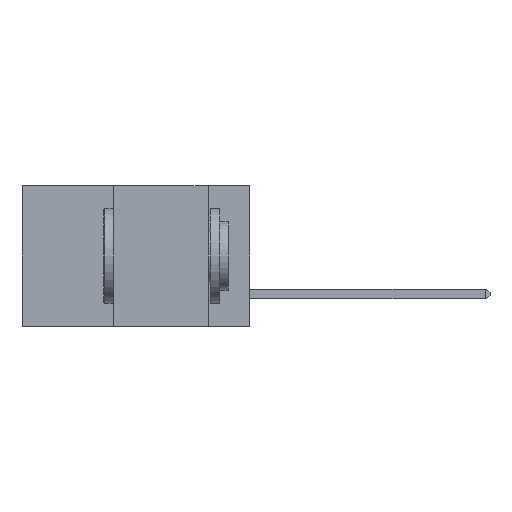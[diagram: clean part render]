
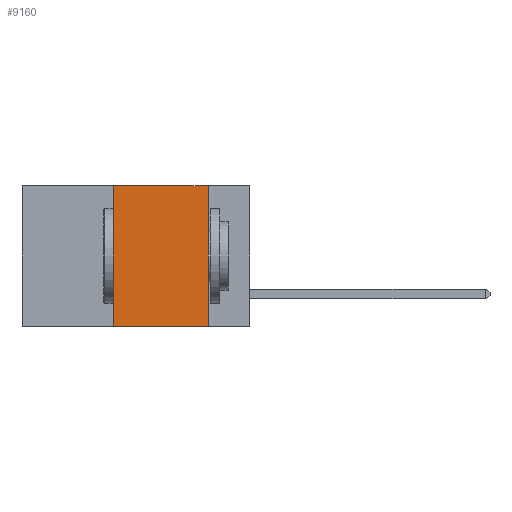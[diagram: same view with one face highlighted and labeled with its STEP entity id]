
A CAD part, left-side view. The second image highlights one B-rep face of the part: STEP entity #9160.
In plain terms, the highlighted planar face has unit normal (-1, 0, 0).
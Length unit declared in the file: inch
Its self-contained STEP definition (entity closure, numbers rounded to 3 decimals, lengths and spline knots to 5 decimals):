
#709 = CARTESIAN_POINT ( 'NONE',  ( 0., 0.6, 0. ) ) ;
#1688 = DIRECTION ( 'NONE',  ( 0., -1., 0. ) ) ;
#2287 = CARTESIAN_POINT ( 'NONE',  ( 0., 0.11, 0. ) ) ;
#3068 = PLANE ( 'NONE',  #20363 ) ;
#3190 = VERTEX_POINT ( 'NONE', #6400 ) ;
#3540 = EDGE_CURVE ( 'NONE', #4156, #19427, #22852, .T. ) ;
#3720 = CARTESIAN_POINT ( 'NONE',  ( 0., 0.11, 0. ) ) ;
#4156 = VERTEX_POINT ( 'NONE', #3720 ) ;
#4837 = LINE ( 'NONE', #22997, #25956 ) ;
#4890 = EDGE_CURVE ( 'NONE', #3190, #4156, #18046, .T. ) ;
#5232 = DIRECTION ( 'NONE',  ( 0., 0., -1. ) ) ;
#6400 = CARTESIAN_POINT ( 'NONE',  ( 0., 0.36, 0. ) ) ;
#6772 = DIRECTION ( 'NONE',  ( 0., -1., 0. ) ) ;
#8476 = ORIENTED_EDGE ( 'NONE', *, *, #3540, .F. ) ;
#8871 = DIRECTION ( 'NONE',  ( 0., 0., 1. ) ) ;
#9160 = ADVANCED_FACE ( 'NONE', ( #16515 ), #3068, .F. ) ;
#10283 = LINE ( 'NONE', #18357, #20376 ) ;
#12125 = VECTOR ( 'NONE', #22815, 39.37008 ) ;
#12218 = CARTESIAN_POINT ( 'NONE',  ( 0., 0.11, -0.37 ) ) ;
#15142 = ORIENTED_EDGE ( 'NONE', *, *, #16748, .F. ) ;
#16515 = FACE_OUTER_BOUND ( 'NONE', #21960, .T. ) ;
#16748 = EDGE_CURVE ( 'NONE', #25343, #3190, #4837, .T. ) ;
#17577 = DIRECTION ( 'NONE',  ( 1., 0., 0. ) ) ;
#17725 = CARTESIAN_POINT ( 'NONE',  ( 0., 0.36, -0.37 ) ) ;
#18046 = LINE ( 'NONE', #23032, #22142 ) ;
#18357 = CARTESIAN_POINT ( 'NONE',  ( 0., 0.6, -0.37 ) ) ;
#19427 = VERTEX_POINT ( 'NONE', #12218 ) ;
#20086 = EDGE_CURVE ( 'NONE', #25343, #19427, #10283, .T. ) ;
#20363 = AXIS2_PLACEMENT_3D ( 'NONE', #709, #17577, #5232 ) ;
#20376 = VECTOR ( 'NONE', #1688, 39.37008 ) ;
#21960 = EDGE_LOOP ( 'NONE', ( #8476, #24621, #15142, #25895 ) ) ;
#22142 = VECTOR ( 'NONE', #6772, 39.37008 ) ;
#22815 = DIRECTION ( 'NONE',  ( 0., 0., -1. ) ) ;
#22852 = LINE ( 'NONE', #2287, #12125 ) ;
#22997 = CARTESIAN_POINT ( 'NONE',  ( 0., 0.36, 0. ) ) ;
#23032 = CARTESIAN_POINT ( 'NONE',  ( 0., 0.6, 0. ) ) ;
#24621 = ORIENTED_EDGE ( 'NONE', *, *, #4890, .F. ) ;
#25343 = VERTEX_POINT ( 'NONE', #17725 ) ;
#25895 = ORIENTED_EDGE ( 'NONE', *, *, #20086, .T. ) ;
#25956 = VECTOR ( 'NONE', #8871, 39.37008 ) ;
